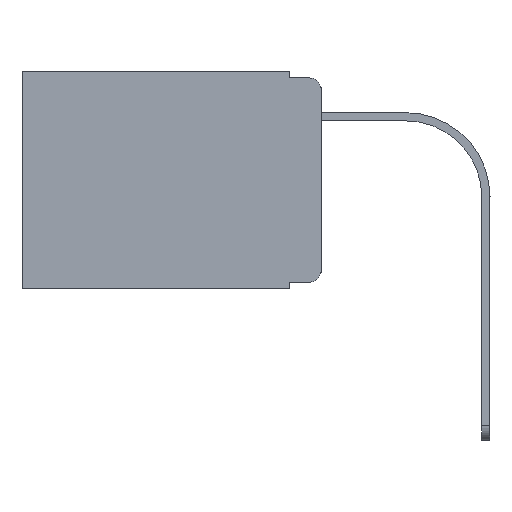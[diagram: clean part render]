
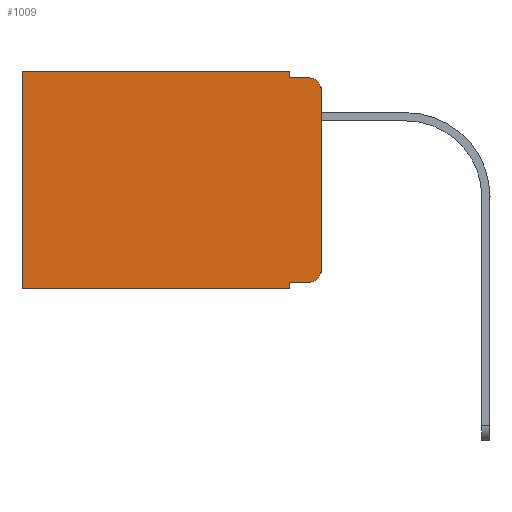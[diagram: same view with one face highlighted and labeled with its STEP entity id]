
A CAD part, left-side view. The second image highlights one B-rep face of the part: STEP entity #1009.
In plain terms, the highlighted planar face has unit normal (-1, 0, 0).
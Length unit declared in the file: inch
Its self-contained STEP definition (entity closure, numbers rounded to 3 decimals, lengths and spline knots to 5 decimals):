
#243 = LINE ( 'NONE', #7229, #857 ) ;
#793 = DIRECTION ( 'NONE',  ( 0., -1., 0. ) ) ;
#816 = ORIENTED_EDGE ( 'NONE', *, *, #2740, .T. ) ;
#857 = VECTOR ( 'NONE', #2975, 39.37008 ) ;
#917 = EDGE_CURVE ( 'NONE', #11351, #10361, #9177, .T. ) ;
#932 = DIRECTION ( 'NONE',  ( 0., 0., -1. ) ) ;
#1009 = ADVANCED_FACE ( 'NONE', ( #9406 ), #7650, .F. ) ;
#1042 = LINE ( 'NONE', #10118, #8263 ) ;
#1544 = DIRECTION ( 'NONE',  ( -1., 0., 0. ) ) ;
#1587 = VECTOR ( 'NONE', #6388, 39.37008 ) ;
#1613 = VECTOR ( 'NONE', #793, 39.37008 ) ;
#1673 = LINE ( 'NONE', #4359, #10989 ) ;
#2339 = CARTESIAN_POINT ( 'NONE',  ( 0.298, 0.473, 0. ) ) ;
#2370 = CIRCLE ( 'NONE', #3700, 0.02 ) ;
#2382 = VERTEX_POINT ( 'NONE', #11396 ) ;
#2392 = DIRECTION ( 'NONE',  ( 0., 0., -1. ) ) ;
#2494 = AXIS2_PLACEMENT_3D ( 'NONE', #2512, #11269, #2392 ) ;
#2512 = CARTESIAN_POINT ( 'NONE',  ( 0.298, 0., 0. ) ) ;
#2740 = EDGE_CURVE ( 'NONE', #11447, #9927, #2370, .T. ) ;
#2896 = CARTESIAN_POINT ( 'NONE',  ( 0.298, 0., 0. ) ) ;
#2975 = DIRECTION ( 'NONE',  ( 0., 1., 0. ) ) ;
#3061 = LINE ( 'NONE', #6563, #11053 ) ;
#3081 = ORIENTED_EDGE ( 'NONE', *, *, #4641, .T. ) ;
#3154 = VERTEX_POINT ( 'NONE', #11149 ) ;
#3164 = CARTESIAN_POINT ( 'NONE',  ( 0.298, 0.051, 0. ) ) ;
#3229 = VERTEX_POINT ( 'NONE', #3164 ) ;
#3332 = CARTESIAN_POINT ( 'NONE',  ( 0.298, 0.051, -0.343 ) ) ;
#3700 = AXIS2_PLACEMENT_3D ( 'NONE', #10305, #7588, #7645 ) ;
#3932 = LINE ( 'NONE', #2896, #1587 ) ;
#4307 = CARTESIAN_POINT ( 'NONE',  ( 0.298, 0.051, -0.333 ) ) ;
#4334 = CARTESIAN_POINT ( 'NONE',  ( 0.298, 0., -0.03 ) ) ;
#4336 = CARTESIAN_POINT ( 'NONE',  ( 0.298, 0.051, -0.333 ) ) ;
#4359 = CARTESIAN_POINT ( 'NONE',  ( 0.298, 0.051, 0. ) ) ;
#4386 = EDGE_CURVE ( 'NONE', #2382, #9927, #3061, .T. ) ;
#4641 = EDGE_CURVE ( 'NONE', #10365, #3154, #6712, .T. ) ;
#4726 = ORIENTED_EDGE ( 'NONE', *, *, #917, .T. ) ;
#5222 = VERTEX_POINT ( 'NONE', #4336 ) ;
#5270 = VECTOR ( 'NONE', #6486, 39.37008 ) ;
#5494 = EDGE_CURVE ( 'NONE', #3229, #2382, #1042, .T. ) ;
#5668 = CARTESIAN_POINT ( 'NONE',  ( 0.298, 0.473, 0. ) ) ;
#5787 = ORIENTED_EDGE ( 'NONE', *, *, #10379, .F. ) ;
#6357 = CARTESIAN_POINT ( 'NONE',  ( 0.298, 0., 0. ) ) ;
#6373 = VERTEX_POINT ( 'NONE', #3332 ) ;
#6383 = ORIENTED_EDGE ( 'NONE', *, *, #5494, .F. ) ;
#6388 = DIRECTION ( 'NONE',  ( 0., 1., 0. ) ) ;
#6445 = EDGE_CURVE ( 'NONE', #11447, #3154, #7342, .T. ) ;
#6463 = CARTESIAN_POINT ( 'NONE',  ( 0.298, 0.02, -0.333 ) ) ;
#6486 = DIRECTION ( 'NONE',  ( 0., 0., -1. ) ) ;
#6563 = CARTESIAN_POINT ( 'NONE',  ( 0.298, 0.051, -0.01 ) ) ;
#6678 = EDGE_CURVE ( 'NONE', #5222, #6373, #1673, .T. ) ;
#6712 = CIRCLE ( 'NONE', #9719, 0.02 ) ;
#6902 = ORIENTED_EDGE ( 'NONE', *, *, #6678, .F. ) ;
#7101 = LINE ( 'NONE', #4307, #1613 ) ;
#7229 = CARTESIAN_POINT ( 'NONE',  ( 0.298, 0., -0.343 ) ) ;
#7293 = DIRECTION ( 'NONE',  ( 0., 0., -1. ) ) ;
#7342 = LINE ( 'NONE', #6357, #11326 ) ;
#7588 = DIRECTION ( 'NONE',  ( -1., 0., 0. ) ) ;
#7645 = DIRECTION ( 'NONE',  ( 0., 0., -1. ) ) ;
#7650 = PLANE ( 'NONE',  #2494 ) ;
#7740 = DIRECTION ( 'NONE',  ( 0., 0., -1. ) ) ;
#7759 = EDGE_LOOP ( 'NONE', ( #9572, #816, #9540, #6383, #10669, #4726, #5787, #6902, #9501, #3081 ) ) ;
#7913 = CARTESIAN_POINT ( 'NONE',  ( 0.298, 0.02, -0.313 ) ) ;
#8263 = VECTOR ( 'NONE', #932, 39.37008 ) ;
#8277 = CARTESIAN_POINT ( 'NONE',  ( 0.298, 0.473, -0.343 ) ) ;
#9177 = LINE ( 'NONE', #5668, #5270 ) ;
#9406 = FACE_OUTER_BOUND ( 'NONE', #7759, .T. ) ;
#9501 = ORIENTED_EDGE ( 'NONE', *, *, #10725, .T. ) ;
#9540 = ORIENTED_EDGE ( 'NONE', *, *, #4386, .F. ) ;
#9572 = ORIENTED_EDGE ( 'NONE', *, *, #6445, .F. ) ;
#9716 = EDGE_CURVE ( 'NONE', #3229, #11351, #3932, .T. ) ;
#9719 = AXIS2_PLACEMENT_3D ( 'NONE', #7913, #1544, #7740 ) ;
#9927 = VERTEX_POINT ( 'NONE', #10299 ) ;
#10118 = CARTESIAN_POINT ( 'NONE',  ( 0.298, 0.051, 0. ) ) ;
#10299 = CARTESIAN_POINT ( 'NONE',  ( 0.298, 0.02, -0.01 ) ) ;
#10305 = CARTESIAN_POINT ( 'NONE',  ( 0.298, 0.02, -0.03 ) ) ;
#10361 = VERTEX_POINT ( 'NONE', #8277 ) ;
#10365 = VERTEX_POINT ( 'NONE', #6463 ) ;
#10379 = EDGE_CURVE ( 'NONE', #6373, #10361, #243, .T. ) ;
#10655 = DIRECTION ( 'NONE',  ( 0., 0., -1. ) ) ;
#10669 = ORIENTED_EDGE ( 'NONE', *, *, #9716, .T. ) ;
#10725 = EDGE_CURVE ( 'NONE', #5222, #10365, #7101, .T. ) ;
#10989 = VECTOR ( 'NONE', #10655, 39.37008 ) ;
#11053 = VECTOR ( 'NONE', #11110, 39.37008 ) ;
#11110 = DIRECTION ( 'NONE',  ( 0., -1., 0. ) ) ;
#11149 = CARTESIAN_POINT ( 'NONE',  ( 0.298, 0., -0.313 ) ) ;
#11269 = DIRECTION ( 'NONE',  ( 1., 0., 0. ) ) ;
#11326 = VECTOR ( 'NONE', #7293, 39.37008 ) ;
#11351 = VERTEX_POINT ( 'NONE', #2339 ) ;
#11396 = CARTESIAN_POINT ( 'NONE',  ( 0.298, 0.051, -0.01 ) ) ;
#11447 = VERTEX_POINT ( 'NONE', #4334 ) ;
